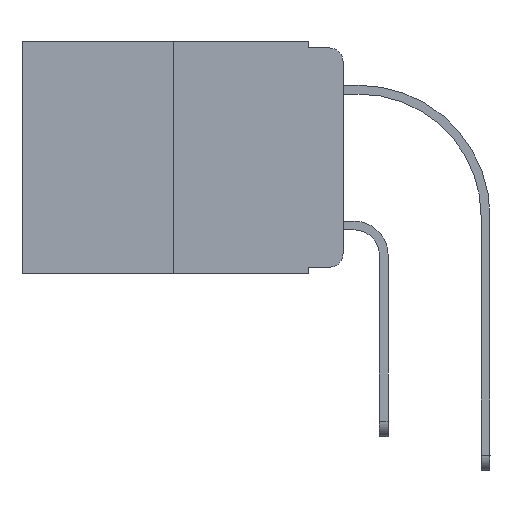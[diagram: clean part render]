
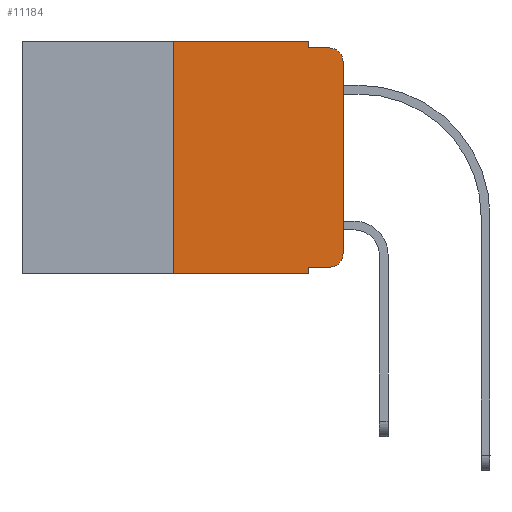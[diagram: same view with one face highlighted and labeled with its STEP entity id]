
A CAD part, left-side view. The second image highlights one B-rep face of the part: STEP entity #11184.
In plain terms, the highlighted planar face has unit normal (-1, 0, 0).
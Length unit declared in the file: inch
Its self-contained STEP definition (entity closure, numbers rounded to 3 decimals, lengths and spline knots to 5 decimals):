
#449 = ORIENTED_EDGE ( 'NONE', *, *, #6086, .T. ) ;
#628 = EDGE_CURVE ( 'NONE', #4228, #10301, #885, .T. ) ;
#873 = ORIENTED_EDGE ( 'NONE', *, *, #23561, .F. ) ;
#885 = LINE ( 'NONE', #3218, #16232 ) ;
#1230 = AXIS2_PLACEMENT_3D ( 'NONE', #20758, #12570, #4019 ) ;
#1270 = LINE ( 'NONE', #18678, #21501 ) ;
#1455 = VERTEX_POINT ( 'NONE', #7663 ) ;
#1741 = ORIENTED_EDGE ( 'NONE', *, *, #5679, .F. ) ;
#1763 = ORIENTED_EDGE ( 'NONE', *, *, #14869, .F. ) ;
#1840 = LINE ( 'NONE', #22450, #6111 ) ;
#2899 = LINE ( 'NONE', #15199, #13167 ) ;
#2964 = VERTEX_POINT ( 'NONE', #6981 ) ;
#3218 = CARTESIAN_POINT ( 'NONE',  ( 0., 0.051, 0. ) ) ;
#3313 = EDGE_CURVE ( 'NONE', #4228, #2964, #21591, .T. ) ;
#4019 = DIRECTION ( 'NONE',  ( 0., 0., -1. ) ) ;
#4228 = VERTEX_POINT ( 'NONE', #27245 ) ;
#4255 = EDGE_CURVE ( 'NONE', #13592, #21989, #8287, .T. ) ;
#4623 = LINE ( 'NONE', #12921, #18958 ) ;
#4861 = DIRECTION ( 'NONE',  ( 0., -1., 0. ) ) ;
#5028 = EDGE_CURVE ( 'NONE', #24480, #21989, #1840, .T. ) ;
#5235 = ORIENTED_EDGE ( 'NONE', *, *, #5028, .F. ) ;
#5679 = EDGE_CURVE ( 'NONE', #21816, #1455, #2899, .T. ) ;
#5757 = ORIENTED_EDGE ( 'NONE', *, *, #3313, .T. ) ;
#5969 = DIRECTION ( 'NONE',  ( 0., -1., 0. ) ) ;
#6086 = EDGE_CURVE ( 'NONE', #21816, #10301, #21267, .T. ) ;
#6111 = VECTOR ( 'NONE', #5969, 39.37008 ) ;
#6309 = ORIENTED_EDGE ( 'NONE', *, *, #628, .F. ) ;
#6439 = EDGE_CURVE ( 'NONE', #24453, #13592, #4623, .T. ) ;
#6967 = CARTESIAN_POINT ( 'NONE',  ( 0., 0.02, -0.01 ) ) ;
#6981 = CARTESIAN_POINT ( 'NONE',  ( 0., 0.02, -0.333 ) ) ;
#7016 = CARTESIAN_POINT ( 'NONE',  ( 0., 0.051, 0. ) ) ;
#7663 = CARTESIAN_POINT ( 'NONE',  ( 0., 0.25, 0. ) ) ;
#7695 = AXIS2_PLACEMENT_3D ( 'NONE', #21311, #21593, #12990 ) ;
#8287 = CIRCLE ( 'NONE', #1230, 0.02 ) ;
#8335 = PLANE ( 'NONE',  #23621 ) ;
#10090 = VECTOR ( 'NONE', #12828, 39.37008 ) ;
#10240 = CARTESIAN_POINT ( 'NONE',  ( 0., 0.051, -0.01 ) ) ;
#10250 = CARTESIAN_POINT ( 'NONE',  ( 0., 0.473, 0. ) ) ;
#10301 = VERTEX_POINT ( 'NONE', #21117 ) ;
#11184 = ADVANCED_FACE ( 'NONE', ( #20775 ), #8335, .F. ) ;
#11337 = DIRECTION ( 'NONE',  ( 0., 0., 1. ) ) ;
#11699 = ORIENTED_EDGE ( 'NONE', *, *, #6439, .T. ) ;
#11766 = DIRECTION ( 'NONE',  ( 0., 0., -1. ) ) ;
#11825 = DIRECTION ( 'NONE',  ( 0., -1., 0. ) ) ;
#12365 = LINE ( 'NONE', #20812, #21912 ) ;
#12457 = DIRECTION ( 'NONE',  ( 1., 0., 0. ) ) ;
#12570 = DIRECTION ( 'NONE',  ( -1., 0., 0. ) ) ;
#12659 = VECTOR ( 'NONE', #4861, 39.37008 ) ;
#12674 = EDGE_LOOP ( 'NONE', ( #11699, #14879, #5235, #1763, #873, #1741, #449, #6309, #5757, #25110 ) ) ;
#12828 = DIRECTION ( 'NONE',  ( 0., -1., 0. ) ) ;
#12921 = CARTESIAN_POINT ( 'NONE',  ( 0., 0., 0. ) ) ;
#12990 = DIRECTION ( 'NONE',  ( 0., 0., -1. ) ) ;
#13167 = VECTOR ( 'NONE', #11337, 39.37008 ) ;
#13592 = VERTEX_POINT ( 'NONE', #22545 ) ;
#14702 = CARTESIAN_POINT ( 'NONE',  ( 0., 0.25, -0.343 ) ) ;
#14869 = EDGE_CURVE ( 'NONE', #17661, #24480, #1270, .T. ) ;
#14879 = ORIENTED_EDGE ( 'NONE', *, *, #4255, .T. ) ;
#15199 = CARTESIAN_POINT ( 'NONE',  ( 0., 0.25, 0. ) ) ;
#16232 = VECTOR ( 'NONE', #24483, 39.37008 ) ;
#17502 = DIRECTION ( 'NONE',  ( 0., 0., 1. ) ) ;
#17621 = CARTESIAN_POINT ( 'NONE',  ( 0., 0., -0.313 ) ) ;
#17661 = VERTEX_POINT ( 'NONE', #7016 ) ;
#18678 = CARTESIAN_POINT ( 'NONE',  ( 0., 0.051, 0. ) ) ;
#18958 = VECTOR ( 'NONE', #17502, 39.37008 ) ;
#19062 = CARTESIAN_POINT ( 'NONE',  ( 0., 0.473, -0.343 ) ) ;
#19646 = CIRCLE ( 'NONE', #7695, 0.02 ) ;
#20758 = CARTESIAN_POINT ( 'NONE',  ( 0., 0.02, -0.03 ) ) ;
#20775 = FACE_OUTER_BOUND ( 'NONE', #12674, .T. ) ;
#20812 = CARTESIAN_POINT ( 'NONE',  ( 0., 0.473, 0. ) ) ;
#21117 = CARTESIAN_POINT ( 'NONE',  ( 0., 0.051, -0.343 ) ) ;
#21187 = DIRECTION ( 'NONE',  ( 0., 0., -1. ) ) ;
#21267 = LINE ( 'NONE', #19062, #10090 ) ;
#21311 = CARTESIAN_POINT ( 'NONE',  ( 0., 0.02, -0.313 ) ) ;
#21501 = VECTOR ( 'NONE', #11766, 39.37008 ) ;
#21591 = LINE ( 'NONE', #22003, #12659 ) ;
#21593 = DIRECTION ( 'NONE',  ( -1., 0., 0. ) ) ;
#21816 = VERTEX_POINT ( 'NONE', #14702 ) ;
#21912 = VECTOR ( 'NONE', #11825, 39.37008 ) ;
#21989 = VERTEX_POINT ( 'NONE', #6967 ) ;
#22003 = CARTESIAN_POINT ( 'NONE',  ( 0., 0.051, -0.333 ) ) ;
#22381 = EDGE_CURVE ( 'NONE', #2964, #24453, #19646, .T. ) ;
#22450 = CARTESIAN_POINT ( 'NONE',  ( 0., 0.051, -0.01 ) ) ;
#22545 = CARTESIAN_POINT ( 'NONE',  ( 0., 0., -0.03 ) ) ;
#23561 = EDGE_CURVE ( 'NONE', #1455, #17661, #12365, .T. ) ;
#23621 = AXIS2_PLACEMENT_3D ( 'NONE', #10250, #12457, #21187 ) ;
#24453 = VERTEX_POINT ( 'NONE', #17621 ) ;
#24480 = VERTEX_POINT ( 'NONE', #10240 ) ;
#24483 = DIRECTION ( 'NONE',  ( 0., 0., -1. ) ) ;
#25110 = ORIENTED_EDGE ( 'NONE', *, *, #22381, .T. ) ;
#27245 = CARTESIAN_POINT ( 'NONE',  ( 0., 0.051, -0.333 ) ) ;
